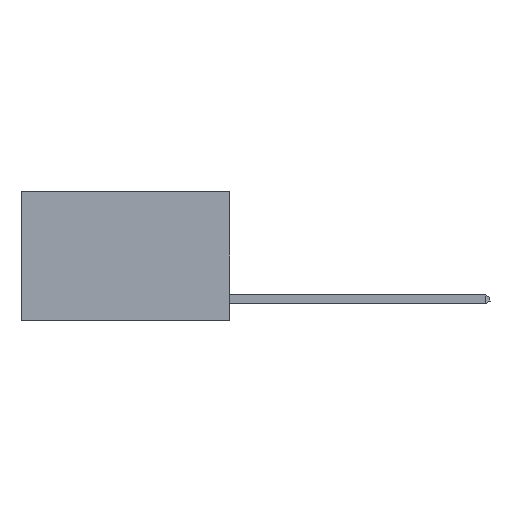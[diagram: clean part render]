
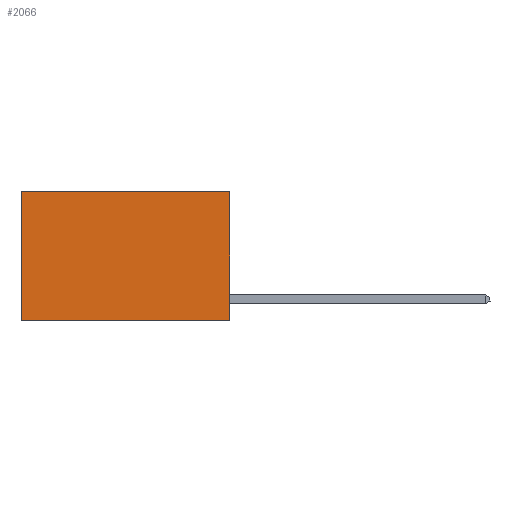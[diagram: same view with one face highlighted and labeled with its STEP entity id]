
A CAD part, left-side view. The second image highlights one B-rep face of the part: STEP entity #2066.
In plain terms, the highlighted planar face has unit normal (-1, 0, 0).
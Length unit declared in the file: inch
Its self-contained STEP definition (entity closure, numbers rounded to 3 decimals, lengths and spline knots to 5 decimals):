
#27 = CARTESIAN_POINT ( 'NONE',  ( 0.2625, 0., -0.37 ) ) ;
#785 = DIRECTION ( 'NONE',  ( 0., 1., 0. ) ) ;
#927 = VECTOR ( 'NONE', #11711, 39.37008 ) ;
#1103 = FACE_OUTER_BOUND ( 'NONE', #10560, .T. ) ;
#1751 = CARTESIAN_POINT ( 'NONE',  ( 0.2625, 0.6, 0. ) ) ;
#2066 = ADVANCED_FACE ( 'NONE', ( #1103 ), #14371, .F. ) ;
#3805 = VERTEX_POINT ( 'NONE', #27 ) ;
#4056 = CARTESIAN_POINT ( 'NONE',  ( 0.2625, 0., 0. ) ) ;
#4171 = VECTOR ( 'NONE', #785, 39.37008 ) ;
#4450 = DIRECTION ( 'NONE',  ( 1., 0., 0. ) ) ;
#4852 = VECTOR ( 'NONE', #14031, 39.37008 ) ;
#5674 = EDGE_CURVE ( 'NONE', #9961, #3805, #13469, .T. ) ;
#5843 = VECTOR ( 'NONE', #17274, 39.37008 ) ;
#6395 = CARTESIAN_POINT ( 'NONE',  ( 0.2625, 0., -0.37 ) ) ;
#7400 = ORIENTED_EDGE ( 'NONE', *, *, #13885, .T. ) ;
#7870 = CARTESIAN_POINT ( 'NONE',  ( 0.2625, 0.6, 0. ) ) ;
#9961 = VERTEX_POINT ( 'NONE', #11786 ) ;
#10140 = EDGE_CURVE ( 'NONE', #3805, #16643, #15566, .T. ) ;
#10560 = EDGE_LOOP ( 'NONE', ( #11599, #17225, #11690, #7400 ) ) ;
#11599 = ORIENTED_EDGE ( 'NONE', *, *, #12090, .T. ) ;
#11690 = ORIENTED_EDGE ( 'NONE', *, *, #5674, .F. ) ;
#11711 = DIRECTION ( 'NONE',  ( 0., 0., -1. ) ) ;
#11786 = CARTESIAN_POINT ( 'NONE',  ( 0.2625, 0., 0. ) ) ;
#11814 = LINE ( 'NONE', #1751, #927 ) ;
#12090 = EDGE_CURVE ( 'NONE', #17938, #16643, #11814, .T. ) ;
#12994 = CARTESIAN_POINT ( 'NONE',  ( 0.2625, 0., 0. ) ) ;
#13469 = LINE ( 'NONE', #15828, #5843 ) ;
#13885 = EDGE_CURVE ( 'NONE', #9961, #17938, #15822, .T. ) ;
#14031 = DIRECTION ( 'NONE',  ( 0., 1., 0. ) ) ;
#14371 = PLANE ( 'NONE',  #14786 ) ;
#14432 = DIRECTION ( 'NONE',  ( 0., 0., -1. ) ) ;
#14449 = CARTESIAN_POINT ( 'NONE',  ( 0.2625, 0.6, -0.37 ) ) ;
#14786 = AXIS2_PLACEMENT_3D ( 'NONE', #12994, #4450, #14432 ) ;
#15566 = LINE ( 'NONE', #6395, #4171 ) ;
#15822 = LINE ( 'NONE', #4056, #4852 ) ;
#15828 = CARTESIAN_POINT ( 'NONE',  ( 0.2625, 0., 0. ) ) ;
#16643 = VERTEX_POINT ( 'NONE', #14449 ) ;
#17225 = ORIENTED_EDGE ( 'NONE', *, *, #10140, .F. ) ;
#17274 = DIRECTION ( 'NONE',  ( 0., 0., -1. ) ) ;
#17938 = VERTEX_POINT ( 'NONE', #7870 ) ;
